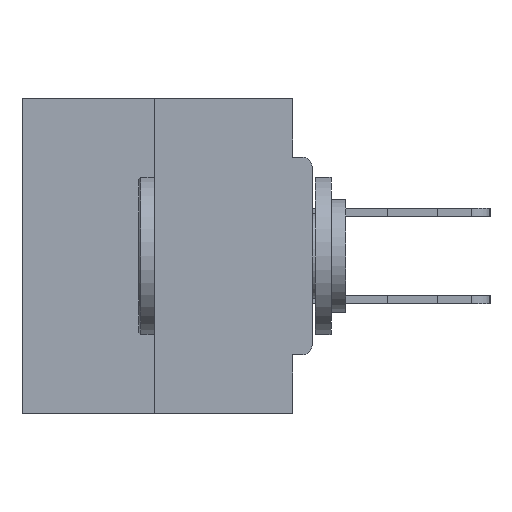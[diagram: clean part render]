
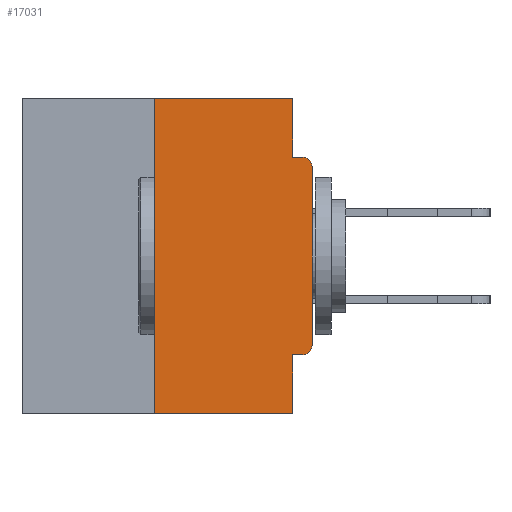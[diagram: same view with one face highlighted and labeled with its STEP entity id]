
A CAD part, left-side view. The second image highlights one B-rep face of the part: STEP entity #17031.
In plain terms, the highlighted planar face has unit normal (-1, 0, 0).
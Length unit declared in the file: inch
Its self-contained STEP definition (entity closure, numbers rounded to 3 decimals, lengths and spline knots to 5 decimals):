
#714 = EDGE_CURVE ( 'NONE', #29235, #18663, #28848, .T. ) ;
#1231 = CARTESIAN_POINT ( 'NONE',  ( 0., 0., -0.1085 ) ) ;
#1261 = DIRECTION ( 'NONE',  ( -1., 0., 0. ) ) ;
#1863 = DIRECTION ( 'NONE',  ( 0., 1., 0. ) ) ;
#3326 = EDGE_LOOP ( 'NONE', ( #27057, #26665, #26508, #17105, #29011, #29891, #35040, #33845, #32219, #10363 ) ) ;
#4355 = DIRECTION ( 'NONE',  ( 0., -1., 0. ) ) ;
#4597 = DIRECTION ( 'NONE',  ( -1., 0., 0. ) ) ;
#4688 = EDGE_CURVE ( 'NONE', #18663, #17728, #19827, .T. ) ;
#4961 = CARTESIAN_POINT ( 'NONE',  ( 0., 0.015, -0.0935 ) ) ;
#5106 = EDGE_CURVE ( 'NONE', #32380, #17728, #18139, .T. ) ;
#5153 = AXIS2_PLACEMENT_3D ( 'NONE', #19874, #1261, #28169 ) ;
#5218 = CARTESIAN_POINT ( 'NONE',  ( 0., 0.031, 0. ) ) ;
#6253 = VECTOR ( 'NONE', #24987, 39.37008 ) ;
#6964 = CARTESIAN_POINT ( 'NONE',  ( 0., 0.015, -0.3915 ) ) ;
#6999 = CARTESIAN_POINT ( 'NONE',  ( 0., 0.031, -0.5 ) ) ;
#7631 = LINE ( 'NONE', #25778, #14824 ) ;
#8033 = EDGE_CURVE ( 'NONE', #16367, #30067, #30733, .T. ) ;
#8197 = LINE ( 'NONE', #17822, #20417 ) ;
#8765 = VECTOR ( 'NONE', #13386, 39.37008 ) ;
#10100 = CARTESIAN_POINT ( 'NONE',  ( 0., 0.25, -0.5 ) ) ;
#10363 = ORIENTED_EDGE ( 'NONE', *, *, #13104, .F. ) ;
#10595 = AXIS2_PLACEMENT_3D ( 'NONE', #6964, #4597, #26087 ) ;
#10645 = CARTESIAN_POINT ( 'NONE',  ( 0., 0.015, -0.4065 ) ) ;
#10793 = VERTEX_POINT ( 'NONE', #34906 ) ;
#11642 = LINE ( 'NONE', #28511, #17140 ) ;
#12327 = DIRECTION ( 'NONE',  ( 0., -1., 0. ) ) ;
#13104 = EDGE_CURVE ( 'NONE', #18955, #32380, #22721, .T. ) ;
#13386 = DIRECTION ( 'NONE',  ( 0., 0., 1. ) ) ;
#13927 = CIRCLE ( 'NONE', #10595, 0.015 ) ;
#14824 = VECTOR ( 'NONE', #12327, 39.37008 ) ;
#15020 = LINE ( 'NONE', #6999, #31501 ) ;
#15679 = EDGE_CURVE ( 'NONE', #21449, #29235, #13927, .T. ) ;
#16367 = VERTEX_POINT ( 'NONE', #10100 ) ;
#16503 = CARTESIAN_POINT ( 'NONE',  ( 0., 0.031, -0.4065 ) ) ;
#17031 = ADVANCED_FACE ( 'NONE', ( #26053 ), #31357, .F. ) ;
#17102 = CARTESIAN_POINT ( 'NONE',  ( 0., 0., 0. ) ) ;
#17105 = ORIENTED_EDGE ( 'NONE', *, *, #18713, .F. ) ;
#17140 = VECTOR ( 'NONE', #1863, 39.37008 ) ;
#17393 = CARTESIAN_POINT ( 'NONE',  ( 0., 0.25, 0. ) ) ;
#17728 = VERTEX_POINT ( 'NONE', #4961 ) ;
#17822 = CARTESIAN_POINT ( 'NONE',  ( 0., 0.46, -0.5 ) ) ;
#18139 = LINE ( 'NONE', #27404, #28252 ) ;
#18663 = VERTEX_POINT ( 'NONE', #1231 ) ;
#18713 = EDGE_CURVE ( 'NONE', #22708, #10793, #15020, .T. ) ;
#18955 = VERTEX_POINT ( 'NONE', #5218 ) ;
#19310 = EDGE_CURVE ( 'NONE', #16367, #10793, #8197, .T. ) ;
#19563 = CARTESIAN_POINT ( 'NONE',  ( 0., 0.031, 0. ) ) ;
#19827 = CIRCLE ( 'NONE', #5153, 0.015 ) ;
#19874 = CARTESIAN_POINT ( 'NONE',  ( 0., 0.015, -0.1085 ) ) ;
#20084 = DIRECTION ( 'NONE',  ( 0., 0., -1. ) ) ;
#20417 = VECTOR ( 'NONE', #4355, 39.37008 ) ;
#21449 = VERTEX_POINT ( 'NONE', #10645 ) ;
#21998 = CARTESIAN_POINT ( 'NONE',  ( 0., 0.031, -0.0935 ) ) ;
#22018 = CARTESIAN_POINT ( 'NONE',  ( 0., 0., -0.3915 ) ) ;
#22284 = DIRECTION ( 'NONE',  ( 0., 0., 1. ) ) ;
#22708 = VERTEX_POINT ( 'NONE', #16503 ) ;
#22721 = LINE ( 'NONE', #19563, #6253 ) ;
#23055 = CARTESIAN_POINT ( 'NONE',  ( 0., 0.46, 0. ) ) ;
#24987 = DIRECTION ( 'NONE',  ( 0., 0., -1. ) ) ;
#25778 = CARTESIAN_POINT ( 'NONE',  ( 0., 0.46, 0. ) ) ;
#26053 = FACE_OUTER_BOUND ( 'NONE', #3326, .T. ) ;
#26087 = DIRECTION ( 'NONE',  ( 0., 0., -1. ) ) ;
#26508 = ORIENTED_EDGE ( 'NONE', *, *, #19310, .T. ) ;
#26665 = ORIENTED_EDGE ( 'NONE', *, *, #8033, .F. ) ;
#27057 = ORIENTED_EDGE ( 'NONE', *, *, #30751, .F. ) ;
#27404 = CARTESIAN_POINT ( 'NONE',  ( 0., 0., -0.0935 ) ) ;
#27645 = EDGE_CURVE ( 'NONE', #21449, #22708, #11642, .T. ) ;
#28169 = DIRECTION ( 'NONE',  ( 0., 0., -1. ) ) ;
#28252 = VECTOR ( 'NONE', #30025, 39.37008 ) ;
#28511 = CARTESIAN_POINT ( 'NONE',  ( 0., 0., -0.4065 ) ) ;
#28848 = LINE ( 'NONE', #17102, #34795 ) ;
#29011 = ORIENTED_EDGE ( 'NONE', *, *, #27645, .F. ) ;
#29235 = VERTEX_POINT ( 'NONE', #22018 ) ;
#29891 = ORIENTED_EDGE ( 'NONE', *, *, #15679, .T. ) ;
#30025 = DIRECTION ( 'NONE',  ( 0., -1., 0. ) ) ;
#30067 = VERTEX_POINT ( 'NONE', #17393 ) ;
#30733 = LINE ( 'NONE', #34681, #8765 ) ;
#30751 = EDGE_CURVE ( 'NONE', #30067, #18955, #7631, .T. ) ;
#31116 = DIRECTION ( 'NONE',  ( 1., 0., 0. ) ) ;
#31357 = PLANE ( 'NONE',  #34429 ) ;
#31501 = VECTOR ( 'NONE', #20084, 39.37008 ) ;
#32219 = ORIENTED_EDGE ( 'NONE', *, *, #5106, .F. ) ;
#32380 = VERTEX_POINT ( 'NONE', #21998 ) ;
#33845 = ORIENTED_EDGE ( 'NONE', *, *, #4688, .T. ) ;
#34085 = DIRECTION ( 'NONE',  ( 0., 0., -1. ) ) ;
#34429 = AXIS2_PLACEMENT_3D ( 'NONE', #23055, #31116, #34085 ) ;
#34681 = CARTESIAN_POINT ( 'NONE',  ( 0., 0.25, 0. ) ) ;
#34795 = VECTOR ( 'NONE', #22284, 39.37008 ) ;
#34906 = CARTESIAN_POINT ( 'NONE',  ( 0., 0.031, -0.5 ) ) ;
#35040 = ORIENTED_EDGE ( 'NONE', *, *, #714, .T. ) ;
